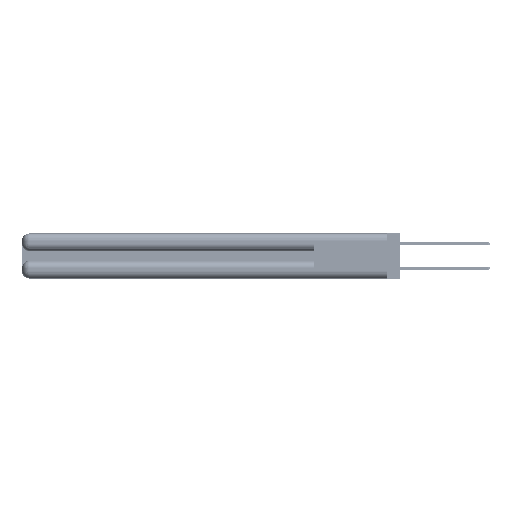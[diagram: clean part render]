
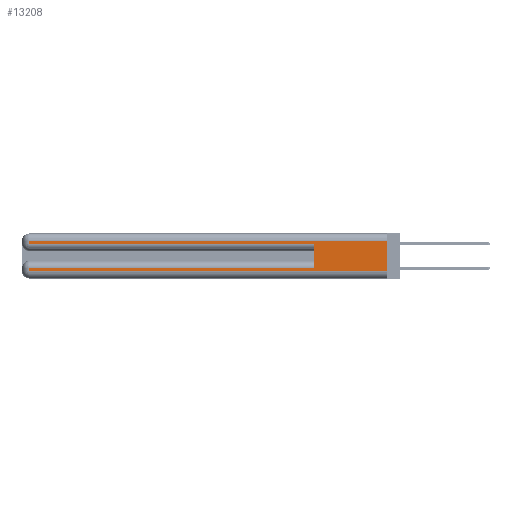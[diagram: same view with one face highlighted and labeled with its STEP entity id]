
A CAD part, left-side view. The second image highlights one B-rep face of the part: STEP entity #13208.
In plain terms, the highlighted planar face has unit normal (-1, 0, 0).
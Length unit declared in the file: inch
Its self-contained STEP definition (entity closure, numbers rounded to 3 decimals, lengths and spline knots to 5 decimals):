
#1728 = VECTOR ( 'NONE', #57067, 39.37008 ) ;
#2755 = LINE ( 'NONE', #29454, #50959 ) ;
#3117 = EDGE_CURVE ( 'NONE', #24394, #45639, #2755, .T. ) ;
#5012 = VECTOR ( 'NONE', #21317, 39.37008 ) ;
#6009 = DIRECTION ( 'NONE',  ( 0., 0., -1. ) ) ;
#7350 = ORIENTED_EDGE ( 'NONE', *, *, #15616, .T. ) ;
#8073 = CARTESIAN_POINT ( 'NONE',  ( 0., 2.94, 0.37 ) ) ;
#8320 = VECTOR ( 'NONE', #34794, 39.37008 ) ;
#8660 = CARTESIAN_POINT ( 'NONE',  ( 0., 0., 0.06 ) ) ;
#9058 = LINE ( 'NONE', #20987, #8320 ) ;
#10054 = CARTESIAN_POINT ( 'NONE',  ( 0., 0., 0.37 ) ) ;
#10172 = CARTESIAN_POINT ( 'NONE',  ( 0., 2.94, 0.06 ) ) ;
#11348 = LINE ( 'NONE', #30099, #5012 ) ;
#12385 = DIRECTION ( 'NONE',  ( 0., 0., -1. ) ) ;
#12605 = EDGE_LOOP ( 'NONE', ( #53595, #49662, #7350, #42695, #52954, #49137, #32228, #44155 ) ) ;
#13208 = ADVANCED_FACE ( 'NONE', ( #52934 ), #19139, .F. ) ;
#14707 = CARTESIAN_POINT ( 'NONE',  ( 0., 2.94, 0.085 ) ) ;
#15616 = EDGE_CURVE ( 'NONE', #52547, #49933, #31758, .T. ) ;
#15783 = CARTESIAN_POINT ( 'NONE',  ( 0., 2.94, 0.31 ) ) ;
#19139 = PLANE ( 'NONE',  #44639 ) ;
#20027 = EDGE_CURVE ( 'NONE', #48700, #37176, #51282, .T. ) ;
#20955 = CARTESIAN_POINT ( 'NONE',  ( 0., 2.94, 0.37 ) ) ;
#20987 = CARTESIAN_POINT ( 'NONE',  ( 0., 0., 0.085 ) ) ;
#21024 = VERTEX_POINT ( 'NONE', #8660 ) ;
#21225 = EDGE_CURVE ( 'NONE', #37176, #21024, #42763, .T. ) ;
#21317 = DIRECTION ( 'NONE',  ( 0., 1., 0. ) ) ;
#22892 = CARTESIAN_POINT ( 'NONE',  ( 0., 0., 0.06 ) ) ;
#24394 = VERTEX_POINT ( 'NONE', #28768 ) ;
#27468 = CARTESIAN_POINT ( 'NONE',  ( 0., 2.94, 0.285 ) ) ;
#28768 = CARTESIAN_POINT ( 'NONE',  ( 0., 0.6, 0.085 ) ) ;
#29249 = DIRECTION ( 'NONE',  ( 0., 0., 1. ) ) ;
#29454 = CARTESIAN_POINT ( 'NONE',  ( 0., 0.6, 0.145 ) ) ;
#30099 = CARTESIAN_POINT ( 'NONE',  ( 0., 0., 0.31 ) ) ;
#31076 = VECTOR ( 'NONE', #12385, 39.37008 ) ;
#31758 = LINE ( 'NONE', #8073, #1728 ) ;
#31933 = CARTESIAN_POINT ( 'NONE',  ( 0., 0., 0.285 ) ) ;
#32228 = ORIENTED_EDGE ( 'NONE', *, *, #20027, .T. ) ;
#34794 = DIRECTION ( 'NONE',  ( 0., 1., 0. ) ) ;
#35131 = CARTESIAN_POINT ( 'NONE',  ( 0., 0.6, 0.285 ) ) ;
#35987 = DIRECTION ( 'NONE',  ( 0., 0., -1. ) ) ;
#36207 = DIRECTION ( 'NONE',  ( 0., -1., 0. ) ) ;
#36820 = EDGE_CURVE ( 'NONE', #24394, #48700, #9058, .T. ) ;
#37176 = VERTEX_POINT ( 'NONE', #10172 ) ;
#39186 = EDGE_CURVE ( 'NONE', #52635, #21024, #53346, .T. ) ;
#40991 = DIRECTION ( 'NONE',  ( 0., -1., 0. ) ) ;
#41134 = DIRECTION ( 'NONE',  ( 1., 0., 0. ) ) ;
#42014 = VECTOR ( 'NONE', #40991, 39.37008 ) ;
#42695 = ORIENTED_EDGE ( 'NONE', *, *, #54307, .T. ) ;
#42763 = LINE ( 'NONE', #22892, #42014 ) ;
#44155 = ORIENTED_EDGE ( 'NONE', *, *, #21225, .T. ) ;
#44639 = AXIS2_PLACEMENT_3D ( 'NONE', #46018, #41134, #6009 ) ;
#44999 = LINE ( 'NONE', #31933, #50618 ) ;
#45548 = EDGE_CURVE ( 'NONE', #52635, #52547, #11348, .T. ) ;
#45639 = VERTEX_POINT ( 'NONE', #35131 ) ;
#46018 = CARTESIAN_POINT ( 'NONE',  ( 0., 0., 0.37 ) ) ;
#48700 = VERTEX_POINT ( 'NONE', #14707 ) ;
#49137 = ORIENTED_EDGE ( 'NONE', *, *, #36820, .T. ) ;
#49662 = ORIENTED_EDGE ( 'NONE', *, *, #45548, .T. ) ;
#49933 = VERTEX_POINT ( 'NONE', #27468 ) ;
#50618 = VECTOR ( 'NONE', #36207, 39.37008 ) ;
#50959 = VECTOR ( 'NONE', #29249, 39.37008 ) ;
#51282 = LINE ( 'NONE', #20955, #31076 ) ;
#52547 = VERTEX_POINT ( 'NONE', #15783 ) ;
#52635 = VERTEX_POINT ( 'NONE', #56333 ) ;
#52934 = FACE_OUTER_BOUND ( 'NONE', #12605, .T. ) ;
#52954 = ORIENTED_EDGE ( 'NONE', *, *, #3117, .F. ) ;
#53346 = LINE ( 'NONE', #10054, #55415 ) ;
#53595 = ORIENTED_EDGE ( 'NONE', *, *, #39186, .F. ) ;
#54307 = EDGE_CURVE ( 'NONE', #49933, #45639, #44999, .T. ) ;
#55415 = VECTOR ( 'NONE', #35987, 39.37008 ) ;
#56333 = CARTESIAN_POINT ( 'NONE',  ( 0., 0., 0.31 ) ) ;
#57067 = DIRECTION ( 'NONE',  ( 0., 0., -1. ) ) ;
